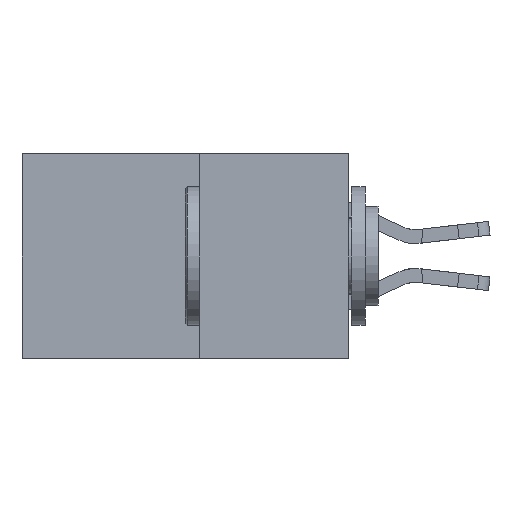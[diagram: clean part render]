
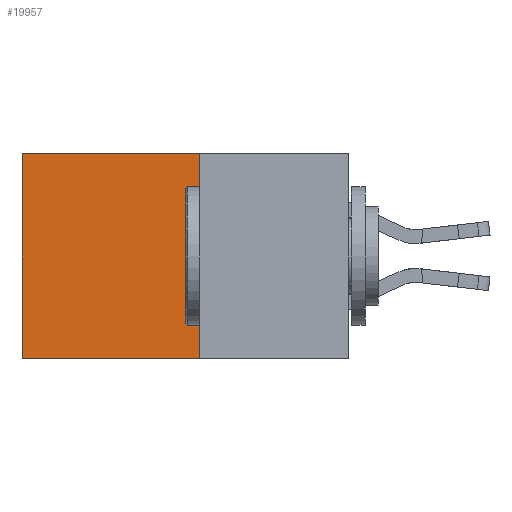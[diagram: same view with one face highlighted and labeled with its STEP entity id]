
A CAD part, left-side view. The second image highlights one B-rep face of the part: STEP entity #19957.
In plain terms, the highlighted planar face has unit normal (-1, 0, 0).
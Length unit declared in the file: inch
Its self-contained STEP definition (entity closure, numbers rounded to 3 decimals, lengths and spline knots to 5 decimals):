
#140 = AXIS2_PLACEMENT_3D ( 'NONE', #22686, #27101, #14467 ) ;
#822 = ORIENTED_EDGE ( 'NONE', *, *, #4293, .F. ) ;
#1452 = VECTOR ( 'NONE', #9924, 39.37008 ) ;
#2679 = VERTEX_POINT ( 'NONE', #26547 ) ;
#3897 = EDGE_CURVE ( 'NONE', #11524, #2679, #15021, .T. ) ;
#4293 = EDGE_CURVE ( 'NONE', #11524, #5712, #5747, .T. ) ;
#4360 = DIRECTION ( 'NONE',  ( 0., 1., 0. ) ) ;
#4391 = CARTESIAN_POINT ( 'NONE',  ( 0.277, 0.27, 0. ) ) ;
#5712 = VERTEX_POINT ( 'NONE', #12413 ) ;
#5747 = LINE ( 'NONE', #9965, #1452 ) ;
#6066 = ORIENTED_EDGE ( 'NONE', *, *, #7489, .T. ) ;
#7489 = EDGE_CURVE ( 'NONE', #2679, #12648, #23698, .T. ) ;
#9915 = EDGE_CURVE ( 'NONE', #5712, #12648, #15741, .T. ) ;
#9924 = DIRECTION ( 'NONE',  ( 0., 0., -1. ) ) ;
#9965 = CARTESIAN_POINT ( 'NONE',  ( 0.277, 0.27, -0.37 ) ) ;
#11238 = CARTESIAN_POINT ( 'NONE',  ( 0.277, 0.59, -0.37 ) ) ;
#11524 = VERTEX_POINT ( 'NONE', #27071 ) ;
#12116 = FACE_OUTER_BOUND ( 'NONE', #17842, .T. ) ;
#12337 = PLANE ( 'NONE',  #140 ) ;
#12413 = CARTESIAN_POINT ( 'NONE',  ( 0.277, 0.27, -0.37 ) ) ;
#12648 = VERTEX_POINT ( 'NONE', #24126 ) ;
#13298 = ORIENTED_EDGE ( 'NONE', *, *, #9915, .F. ) ;
#13353 = DIRECTION ( 'NONE',  ( 0., 0., -1. ) ) ;
#14467 = DIRECTION ( 'NONE',  ( 0., 0., -1. ) ) ;
#15021 = LINE ( 'NONE', #4391, #25563 ) ;
#15439 = ORIENTED_EDGE ( 'NONE', *, *, #3897, .T. ) ;
#15741 = LINE ( 'NONE', #24347, #25636 ) ;
#15980 = DIRECTION ( 'NONE',  ( 0., 1., 0. ) ) ;
#17842 = EDGE_LOOP ( 'NONE', ( #6066, #13298, #822, #15439 ) ) ;
#19957 = ADVANCED_FACE ( 'NONE', ( #12116 ), #12337, .F. ) ;
#22686 = CARTESIAN_POINT ( 'NONE',  ( 0.277, 0.27, -0.37 ) ) ;
#23010 = VECTOR ( 'NONE', #13353, 39.37008 ) ;
#23698 = LINE ( 'NONE', #11238, #23010 ) ;
#24126 = CARTESIAN_POINT ( 'NONE',  ( 0.277, 0.59, -0.37 ) ) ;
#24347 = CARTESIAN_POINT ( 'NONE',  ( 0.277, 0.27, -0.37 ) ) ;
#25563 = VECTOR ( 'NONE', #4360, 39.37008 ) ;
#25636 = VECTOR ( 'NONE', #15980, 39.37008 ) ;
#26547 = CARTESIAN_POINT ( 'NONE',  ( 0.277, 0.59, 0. ) ) ;
#27071 = CARTESIAN_POINT ( 'NONE',  ( 0.277, 0.27, 0. ) ) ;
#27101 = DIRECTION ( 'NONE',  ( 1., 0., 0. ) ) ;
